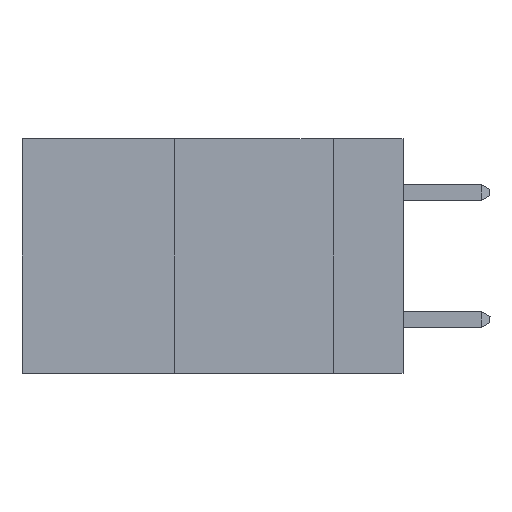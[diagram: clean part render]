
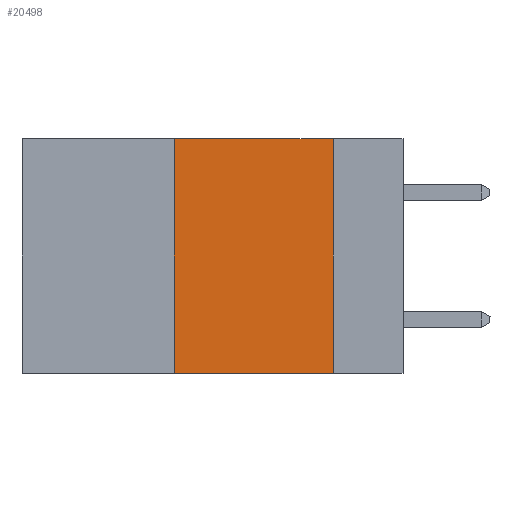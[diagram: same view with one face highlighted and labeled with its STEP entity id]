
A CAD part, left-side view. The second image highlights one B-rep face of the part: STEP entity #20498.
In plain terms, the highlighted planar face has unit normal (-1, 0, 0).
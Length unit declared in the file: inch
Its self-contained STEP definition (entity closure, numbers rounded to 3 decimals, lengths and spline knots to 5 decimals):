
#275 = PLANE ( 'NONE',  #7029 ) ;
#1613 = LINE ( 'NONE', #11454, #4170 ) ;
#3385 = VERTEX_POINT ( 'NONE', #14029 ) ;
#3805 = VERTEX_POINT ( 'NONE', #9777 ) ;
#3823 = VECTOR ( 'NONE', #16458, 39.37008 ) ;
#4170 = VECTOR ( 'NONE', #22280, 39.37008 ) ;
#4447 = CARTESIAN_POINT ( 'NONE',  ( 0., 0.36, 0. ) ) ;
#4649 = ORIENTED_EDGE ( 'NONE', *, *, #13413, .F. ) ;
#5202 = CARTESIAN_POINT ( 'NONE',  ( 0., 0.6, 0. ) ) ;
#5556 = EDGE_LOOP ( 'NONE', ( #21962, #21430, #4649, #20059 ) ) ;
#5942 = EDGE_CURVE ( 'NONE', #3805, #21109, #6292, .T. ) ;
#6292 = LINE ( 'NONE', #15425, #8256 ) ;
#7029 = AXIS2_PLACEMENT_3D ( 'NONE', #5202, #14203, #7561 ) ;
#7561 = DIRECTION ( 'NONE',  ( 0., 0., -1. ) ) ;
#8256 = VECTOR ( 'NONE', #17445, 39.37008 ) ;
#9003 = VERTEX_POINT ( 'NONE', #4447 ) ;
#9204 = EDGE_CURVE ( 'NONE', #3385, #21109, #1613, .T. ) ;
#9591 = DIRECTION ( 'NONE',  ( 0., 0., 1. ) ) ;
#9777 = CARTESIAN_POINT ( 'NONE',  ( 0., 0.11, 0. ) ) ;
#10961 = LINE ( 'NONE', #12629, #3823 ) ;
#11125 = CARTESIAN_POINT ( 'NONE',  ( 0., 0.36, 0. ) ) ;
#11454 = CARTESIAN_POINT ( 'NONE',  ( 0., 0.6, -0.37 ) ) ;
#11887 = CARTESIAN_POINT ( 'NONE',  ( 0., 0.11, -0.37 ) ) ;
#12466 = FACE_OUTER_BOUND ( 'NONE', #5556, .T. ) ;
#12629 = CARTESIAN_POINT ( 'NONE',  ( 0., 0.6, 0. ) ) ;
#13413 = EDGE_CURVE ( 'NONE', #3385, #9003, #23172, .T. ) ;
#13652 = VECTOR ( 'NONE', #9591, 39.37008 ) ;
#14029 = CARTESIAN_POINT ( 'NONE',  ( 0., 0.36, -0.37 ) ) ;
#14203 = DIRECTION ( 'NONE',  ( 1., 0., 0. ) ) ;
#15425 = CARTESIAN_POINT ( 'NONE',  ( 0., 0.11, 0. ) ) ;
#15984 = EDGE_CURVE ( 'NONE', #9003, #3805, #10961, .T. ) ;
#16458 = DIRECTION ( 'NONE',  ( 0., -1., 0. ) ) ;
#17445 = DIRECTION ( 'NONE',  ( 0., 0., -1. ) ) ;
#20059 = ORIENTED_EDGE ( 'NONE', *, *, #9204, .T. ) ;
#20498 = ADVANCED_FACE ( 'NONE', ( #12466 ), #275, .F. ) ;
#21109 = VERTEX_POINT ( 'NONE', #11887 ) ;
#21430 = ORIENTED_EDGE ( 'NONE', *, *, #15984, .F. ) ;
#21962 = ORIENTED_EDGE ( 'NONE', *, *, #5942, .F. ) ;
#22280 = DIRECTION ( 'NONE',  ( 0., -1., 0. ) ) ;
#23172 = LINE ( 'NONE', #11125, #13652 ) ;
